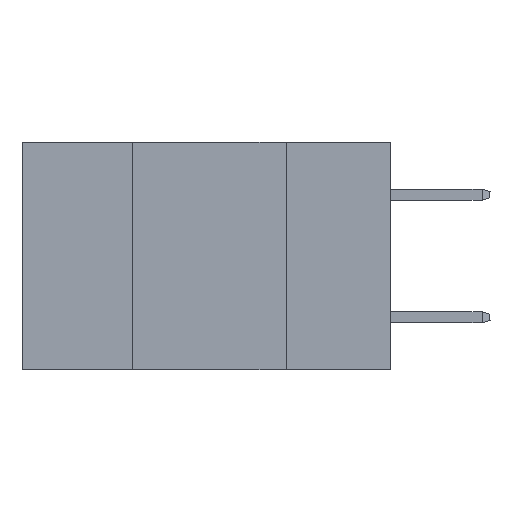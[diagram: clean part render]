
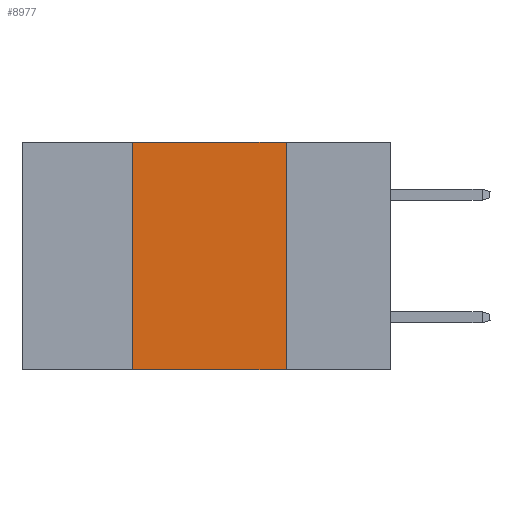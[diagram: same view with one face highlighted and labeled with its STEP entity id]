
A CAD part, left-side view. The second image highlights one B-rep face of the part: STEP entity #8977.
In plain terms, the highlighted planar face has unit normal (-1, 0, 0).
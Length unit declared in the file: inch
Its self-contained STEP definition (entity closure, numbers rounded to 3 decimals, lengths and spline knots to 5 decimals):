
#101 = EDGE_CURVE ( 'NONE', #20055, #5720, #2897, .T. ) ;
#1433 = PLANE ( 'NONE',  #8347 ) ;
#1934 = CARTESIAN_POINT ( 'NONE',  ( 0., 0.6, 0. ) ) ;
#2897 = LINE ( 'NONE', #30905, #34034 ) ;
#5720 = VERTEX_POINT ( 'NONE', #35940 ) ;
#6140 = VECTOR ( 'NONE', #21883, 39.37008 ) ;
#6320 = VERTEX_POINT ( 'NONE', #31317 ) ;
#8347 = AXIS2_PLACEMENT_3D ( 'NONE', #1934, #14462, #10794 ) ;
#8618 = LINE ( 'NONE', #12411, #26143 ) ;
#8977 = ADVANCED_FACE ( 'NONE', ( #20891 ), #1433, .F. ) ;
#9396 = DIRECTION ( 'NONE',  ( 0., -1., 0. ) ) ;
#9896 = ORIENTED_EDGE ( 'NONE', *, *, #31114, .F. ) ;
#10273 = VERTEX_POINT ( 'NONE', #14379 ) ;
#10693 = ORIENTED_EDGE ( 'NONE', *, *, #19734, .T. ) ;
#10794 = DIRECTION ( 'NONE',  ( 0., 0., -1. ) ) ;
#12411 = CARTESIAN_POINT ( 'NONE',  ( 0., 0.6, 0. ) ) ;
#14379 = CARTESIAN_POINT ( 'NONE',  ( 0., 0.42, 0. ) ) ;
#14462 = DIRECTION ( 'NONE',  ( 1., 0., 0. ) ) ;
#14879 = LINE ( 'NONE', #30743, #6140 ) ;
#19734 = EDGE_CURVE ( 'NONE', #6320, #5720, #37668, .T. ) ;
#20055 = VERTEX_POINT ( 'NONE', #37627 ) ;
#20891 = FACE_OUTER_BOUND ( 'NONE', #31606, .T. ) ;
#21563 = VECTOR ( 'NONE', #26805, 39.37008 ) ;
#21883 = DIRECTION ( 'NONE',  ( 0., 0., 1. ) ) ;
#21922 = ORIENTED_EDGE ( 'NONE', *, *, #22578, .F. ) ;
#22578 = EDGE_CURVE ( 'NONE', #6320, #10273, #14879, .T. ) ;
#26143 = VECTOR ( 'NONE', #9396, 39.37008 ) ;
#26805 = DIRECTION ( 'NONE',  ( 0., -1., 0. ) ) ;
#27075 = CARTESIAN_POINT ( 'NONE',  ( 0., 0.6, -0.37 ) ) ;
#30501 = DIRECTION ( 'NONE',  ( 0., 0., -1. ) ) ;
#30743 = CARTESIAN_POINT ( 'NONE',  ( 0., 0.42, 0. ) ) ;
#30905 = CARTESIAN_POINT ( 'NONE',  ( 0., 0.17, 0. ) ) ;
#31114 = EDGE_CURVE ( 'NONE', #10273, #20055, #8618, .T. ) ;
#31317 = CARTESIAN_POINT ( 'NONE',  ( 0., 0.42, -0.37 ) ) ;
#31606 = EDGE_LOOP ( 'NONE', ( #39592, #9896, #21922, #10693 ) ) ;
#34034 = VECTOR ( 'NONE', #30501, 39.37008 ) ;
#35940 = CARTESIAN_POINT ( 'NONE',  ( 0., 0.17, -0.37 ) ) ;
#37627 = CARTESIAN_POINT ( 'NONE',  ( 0., 0.17, 0. ) ) ;
#37668 = LINE ( 'NONE', #27075, #21563 ) ;
#39592 = ORIENTED_EDGE ( 'NONE', *, *, #101, .F. ) ;
